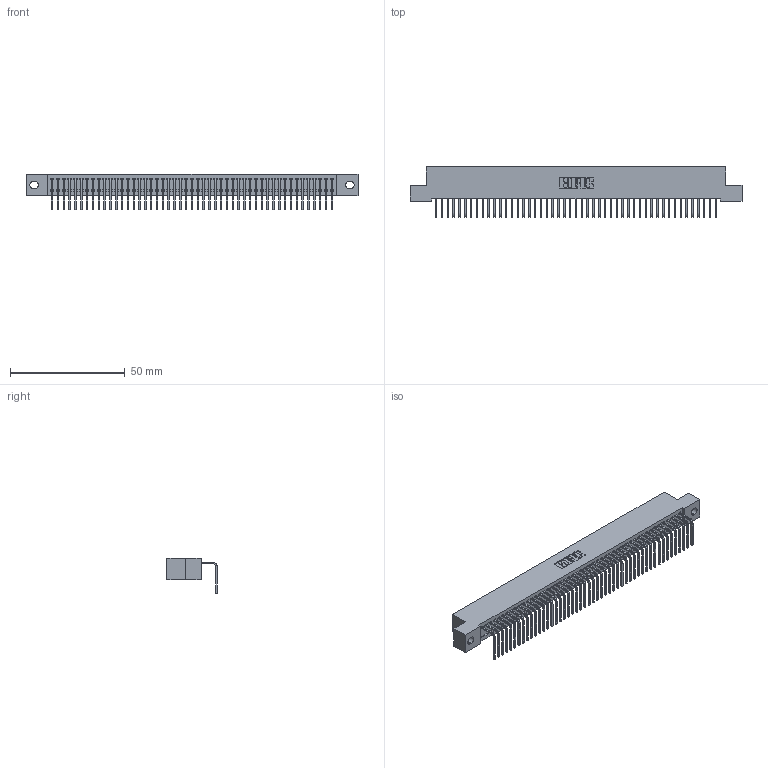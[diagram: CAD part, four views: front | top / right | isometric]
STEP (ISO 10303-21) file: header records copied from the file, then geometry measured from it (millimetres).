
FILE_DESCRIPTION (( 'STEP AP203' ), '1' );
FILE_NAME ('392-049-558-102.STEP', '2019-10-08T10:58:10', ( '' ), ( '' ), 'SwSTEP 2.0', 'SolidWorks 2016', '' );
FILE_SCHEMA (( 'CONFIG_CONTROL_DESIGN' ));
Length unit declared in the file: inch
Products named in the file (3): 345-292-001_558 Tail - 2; 392-049-558-102; 342 Part_.128 Slot
Assembly tree (50 placements, depth 2):
  392-049-558-102
    342 Part_.128 Slot
    345-292-001_558 Tail - 2  x49
Bounding box: 144.78 x 21.91 x 15.62 mm (x, y, z)
Volume: 12831.2 mm3; surface area: 19659.6 mm2
Topology: 50 solids, 50 shells, 3054 faces, 9229 edges, 6086 vertices
Faces by surface type: plane 2226, cylinder 828
Entity records: 29137 total; most frequent: CARTESIAN_POINT 5033, ORIENTED_EDGE 5018, DIRECTION 4231, EDGE_CURVE 2509, LINE 2381, VECTOR 2381, VERTEX_POINT 1670, AXIS2_PLACEMENT_3D 925
